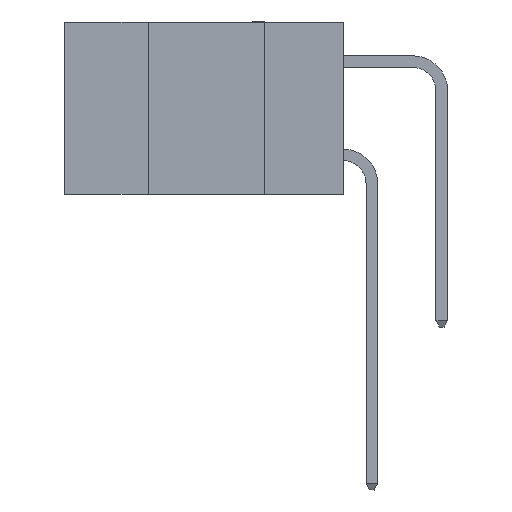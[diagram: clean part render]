
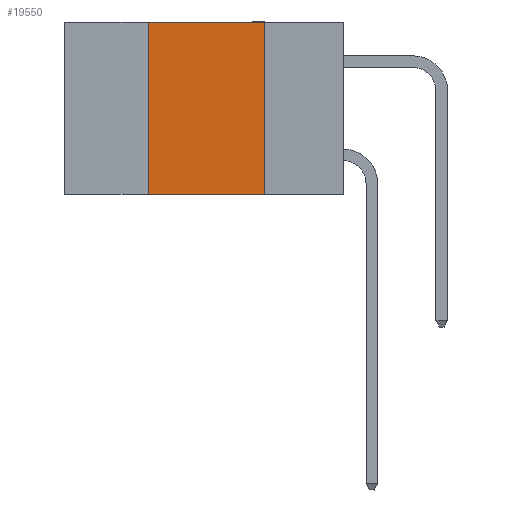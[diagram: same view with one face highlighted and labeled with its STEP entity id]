
A CAD part, left-side view. The second image highlights one B-rep face of the part: STEP entity #19550.
In plain terms, the highlighted planar face has unit normal (-1, 0, 0).
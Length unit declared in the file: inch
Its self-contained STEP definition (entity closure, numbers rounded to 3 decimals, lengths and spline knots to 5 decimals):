
#1111 = ORIENTED_EDGE ( 'NONE', *, *, #8716, .F. ) ;
#1230 = CARTESIAN_POINT ( 'NONE',  ( 0., 0.17, -0.37 ) ) ;
#1448 = CARTESIAN_POINT ( 'NONE',  ( 0., 0.17, 0. ) ) ;
#1564 = EDGE_CURVE ( 'NONE', #17394, #14150, #19232, .T. ) ;
#4880 = ORIENTED_EDGE ( 'NONE', *, *, #1564, .F. ) ;
#5290 = DIRECTION ( 'NONE',  ( 0., -1., 0. ) ) ;
#5982 = ORIENTED_EDGE ( 'NONE', *, *, #5999, .T. ) ;
#5999 = EDGE_CURVE ( 'NONE', #12058, #6932, #9351, .T. ) ;
#6900 = VECTOR ( 'NONE', #13944, 39.37008 ) ;
#6932 = VERTEX_POINT ( 'NONE', #1230 ) ;
#8030 = LINE ( 'NONE', #22927, #6900 ) ;
#8716 = EDGE_CURVE ( 'NONE', #12058, #17394, #11505, .T. ) ;
#9122 = FACE_OUTER_BOUND ( 'NONE', #15415, .T. ) ;
#9225 = DIRECTION ( 'NONE',  ( 1., 0., 0. ) ) ;
#9351 = LINE ( 'NONE', #15907, #18468 ) ;
#11505 = LINE ( 'NONE', #11771, #21218 ) ;
#11771 = CARTESIAN_POINT ( 'NONE',  ( 0., 0.42, 0. ) ) ;
#12058 = VERTEX_POINT ( 'NONE', #14214 ) ;
#13944 = DIRECTION ( 'NONE',  ( 0., 0., -1. ) ) ;
#13962 = ORIENTED_EDGE ( 'NONE', *, *, #15360, .F. ) ;
#14150 = VERTEX_POINT ( 'NONE', #1448 ) ;
#14214 = CARTESIAN_POINT ( 'NONE',  ( 0., 0.42, -0.37 ) ) ;
#14296 = CARTESIAN_POINT ( 'NONE',  ( 0., 0.42, 0. ) ) ;
#14369 = VECTOR ( 'NONE', #15177, 39.37008 ) ;
#14708 = CARTESIAN_POINT ( 'NONE',  ( 0., 0.6, 0. ) ) ;
#15169 = CARTESIAN_POINT ( 'NONE',  ( 0., 0.6, 0. ) ) ;
#15177 = DIRECTION ( 'NONE',  ( 0., -1., 0. ) ) ;
#15360 = EDGE_CURVE ( 'NONE', #14150, #6932, #8030, .T. ) ;
#15415 = EDGE_LOOP ( 'NONE', ( #13962, #4880, #1111, #5982 ) ) ;
#15907 = CARTESIAN_POINT ( 'NONE',  ( 0., 0.6, -0.37 ) ) ;
#16564 = PLANE ( 'NONE',  #19946 ) ;
#17394 = VERTEX_POINT ( 'NONE', #14296 ) ;
#18374 = DIRECTION ( 'NONE',  ( 0., 0., -1. ) ) ;
#18468 = VECTOR ( 'NONE', #5290, 39.37008 ) ;
#19232 = LINE ( 'NONE', #15169, #14369 ) ;
#19550 = ADVANCED_FACE ( 'NONE', ( #9122 ), #16564, .F. ) ;
#19946 = AXIS2_PLACEMENT_3D ( 'NONE', #14708, #9225, #18374 ) ;
#21218 = VECTOR ( 'NONE', #22222, 39.37008 ) ;
#22222 = DIRECTION ( 'NONE',  ( 0., 0., 1. ) ) ;
#22927 = CARTESIAN_POINT ( 'NONE',  ( 0., 0.17, 0. ) ) ;
